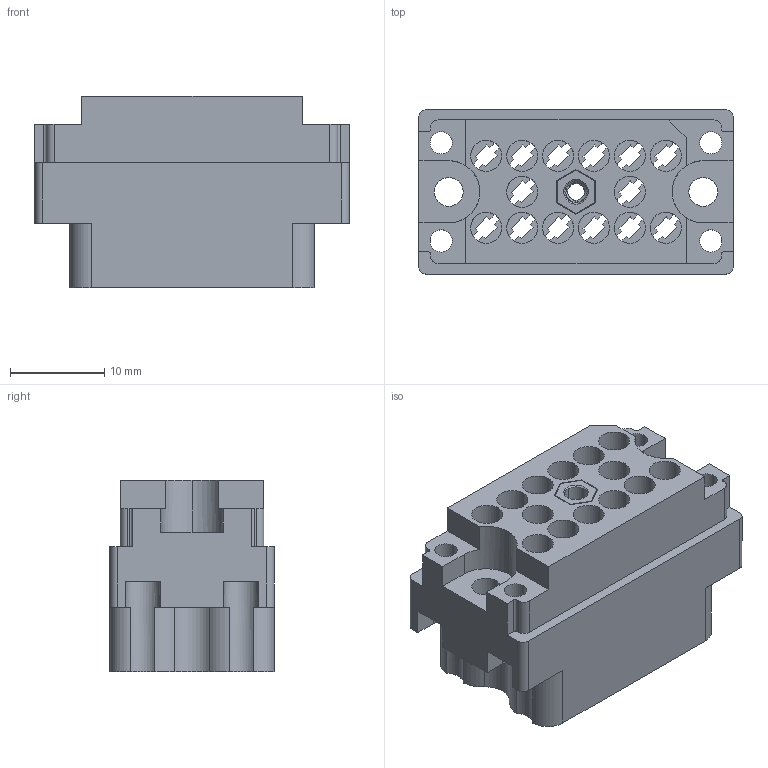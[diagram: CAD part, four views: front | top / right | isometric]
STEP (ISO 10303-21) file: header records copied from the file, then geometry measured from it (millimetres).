
FILE_DESCRIPTION (( 'STEP AP203' ), '1' );
FILE_NAME ('519-014-000-306.STEP', '2020-03-02T19:32:04', ( '' ), ( '' ), 'SwSTEP 2.0', 'SolidWorks 2016', '' );
FILE_SCHEMA (( 'CONFIG_CONTROL_DESIGN' ));
Length unit declared in the file: inch
Products named in the file (3): 519 Plug Insulator_014; 519-014-000-306; 516-252-025-100_516-252-025-100
Assembly tree (2 placements, depth 2):
  519-014-000-306
    519 Plug Insulator_014
    516-252-025-100_516-252-025-100
Bounding box: 33.32 x 17.42 x 20.27 mm (x, y, z)
Volume: 5012 mm3; surface area: 6361 mm2
Topology: 2 solids, 2 shells, 550 faces, 1592 edges, 1057 vertices
Faces by surface type: plane 338, cylinder 198, cone 11, bspline 3
Entity records: 21065 total; most frequent: CARTESIAN_POINT 5920, ORIENTED_EDGE 3184, DIRECTION 3067, EDGE_CURVE 1592, VECTOR 1109, LINE 1109, VERTEX_POINT 1057, AXIS2_PLACEMENT_3D 979
